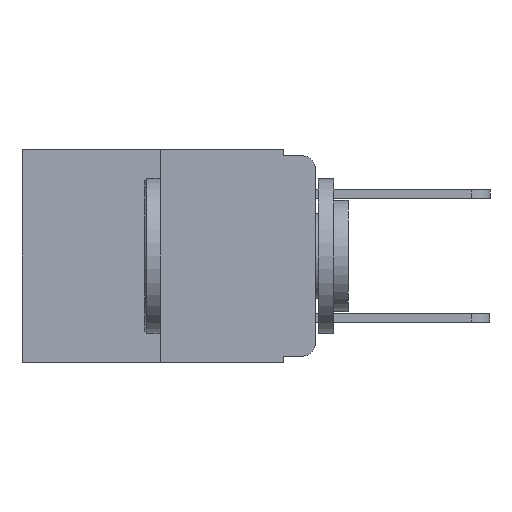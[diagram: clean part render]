
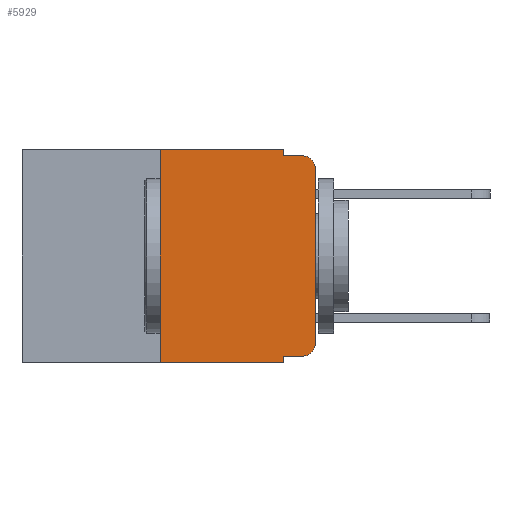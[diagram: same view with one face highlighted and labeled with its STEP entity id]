
A CAD part, left-side view. The second image highlights one B-rep face of the part: STEP entity #5929.
In plain terms, the highlighted planar face has unit normal (-1, 0, 0).
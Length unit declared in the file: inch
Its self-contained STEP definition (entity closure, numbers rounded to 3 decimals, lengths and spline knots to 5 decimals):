
#421 = EDGE_CURVE ( 'NONE', #12266, #12608, #3539, .T. ) ;
#1269 = CIRCLE ( 'NONE', #4434, 0.02 ) ;
#1319 = EDGE_CURVE ( 'NONE', #3115, #10111, #10894, .T. ) ;
#1534 = CARTESIAN_POINT ( 'NONE',  ( 0., 0.02, -0.01 ) ) ;
#1703 = VERTEX_POINT ( 'NONE', #7854 ) ;
#1953 = VECTOR ( 'NONE', #9794, 39.37008 ) ;
#2474 = DIRECTION ( 'NONE',  ( 0., 0., 1. ) ) ;
#2900 = CARTESIAN_POINT ( 'NONE',  ( 0., 0.25, -0.343 ) ) ;
#3115 = VERTEX_POINT ( 'NONE', #11257 ) ;
#3539 = LINE ( 'NONE', #11785, #9305 ) ;
#4050 = CARTESIAN_POINT ( 'NONE',  ( 0., 0.051, -0.333 ) ) ;
#4121 = VECTOR ( 'NONE', #14405, 39.37008 ) ;
#4192 = VERTEX_POINT ( 'NONE', #7693 ) ;
#4434 = AXIS2_PLACEMENT_3D ( 'NONE', #6604, #14104, #13889 ) ;
#4486 = EDGE_CURVE ( 'NONE', #14955, #12266, #11818, .T. ) ;
#5075 = DIRECTION ( 'NONE',  ( 0., 0., -1. ) ) ;
#5216 = EDGE_CURVE ( 'NONE', #6627, #4192, #1269, .T. ) ;
#5263 = EDGE_CURVE ( 'NONE', #14955, #1703, #9962, .T. ) ;
#5427 = DIRECTION ( 'NONE',  ( 0., -1., 0. ) ) ;
#5702 = LINE ( 'NONE', #11659, #8045 ) ;
#5869 = EDGE_CURVE ( 'NONE', #12608, #3115, #8305, .T. ) ;
#5929 = ADVANCED_FACE ( 'NONE', ( #10449 ), #9889, .F. ) ;
#6332 = CIRCLE ( 'NONE', #6473, 0.02 ) ;
#6473 = AXIS2_PLACEMENT_3D ( 'NONE', #7149, #14585, #8295 ) ;
#6604 = CARTESIAN_POINT ( 'NONE',  ( 0., 0.02, -0.313 ) ) ;
#6627 = VERTEX_POINT ( 'NONE', #7120 ) ;
#6712 = CARTESIAN_POINT ( 'NONE',  ( 0., 0.473, -0.343 ) ) ;
#7092 = CARTESIAN_POINT ( 'NONE',  ( 0., 0.25, 0. ) ) ;
#7120 = CARTESIAN_POINT ( 'NONE',  ( 0., 0.02, -0.333 ) ) ;
#7149 = CARTESIAN_POINT ( 'NONE',  ( 0., 0.02, -0.03 ) ) ;
#7528 = CARTESIAN_POINT ( 'NONE',  ( 0., 0.473, 0. ) ) ;
#7693 = CARTESIAN_POINT ( 'NONE',  ( 0., 0., -0.313 ) ) ;
#7854 = CARTESIAN_POINT ( 'NONE',  ( 0., 0.051, -0.343 ) ) ;
#7859 = DIRECTION ( 'NONE',  ( 0., -1., 0. ) ) ;
#8045 = VECTOR ( 'NONE', #5075, 39.37008 ) ;
#8229 = EDGE_CURVE ( 'NONE', #4192, #14223, #12916, .T. ) ;
#8295 = DIRECTION ( 'NONE',  ( 0., 0., -1. ) ) ;
#8305 = LINE ( 'NONE', #13317, #1953 ) ;
#8575 = DIRECTION ( 'NONE',  ( 0., -1., 0. ) ) ;
#8607 = CARTESIAN_POINT ( 'NONE',  ( 0., 0.051, -0.01 ) ) ;
#8660 = VECTOR ( 'NONE', #2474, 39.37008 ) ;
#8827 = CARTESIAN_POINT ( 'NONE',  ( 0., 0.051, -0.333 ) ) ;
#9305 = VECTOR ( 'NONE', #5427, 39.37008 ) ;
#9314 = ORIENTED_EDGE ( 'NONE', *, *, #8229, .T. ) ;
#9353 = VECTOR ( 'NONE', #14069, 39.37008 ) ;
#9794 = DIRECTION ( 'NONE',  ( 0., 0., -1. ) ) ;
#9889 = PLANE ( 'NONE',  #14348 ) ;
#9961 = EDGE_CURVE ( 'NONE', #14886, #1703, #5702, .T. ) ;
#9962 = LINE ( 'NONE', #6712, #12493 ) ;
#10006 = CARTESIAN_POINT ( 'NONE',  ( 0., 0.25, 0. ) ) ;
#10054 = ORIENTED_EDGE ( 'NONE', *, *, #13132, .T. ) ;
#10107 = ORIENTED_EDGE ( 'NONE', *, *, #1319, .F. ) ;
#10111 = VERTEX_POINT ( 'NONE', #1534 ) ;
#10449 = FACE_OUTER_BOUND ( 'NONE', #10638, .T. ) ;
#10560 = VECTOR ( 'NONE', #8575, 39.37008 ) ;
#10638 = EDGE_LOOP ( 'NONE', ( #9314, #10054, #10107, #11231, #11241, #11255, #11309, #11341, #11711, #11885 ) ) ;
#10894 = LINE ( 'NONE', #8607, #10560 ) ;
#11231 = ORIENTED_EDGE ( 'NONE', *, *, #5869, .F. ) ;
#11241 = ORIENTED_EDGE ( 'NONE', *, *, #421, .F. ) ;
#11255 = ORIENTED_EDGE ( 'NONE', *, *, #4486, .F. ) ;
#11257 = CARTESIAN_POINT ( 'NONE',  ( 0., 0.051, -0.01 ) ) ;
#11309 = ORIENTED_EDGE ( 'NONE', *, *, #5263, .T. ) ;
#11341 = ORIENTED_EDGE ( 'NONE', *, *, #9961, .F. ) ;
#11502 = CARTESIAN_POINT ( 'NONE',  ( 0., 0.051, 0. ) ) ;
#11659 = CARTESIAN_POINT ( 'NONE',  ( 0., 0.051, 0. ) ) ;
#11711 = ORIENTED_EDGE ( 'NONE', *, *, #12145, .T. ) ;
#11785 = CARTESIAN_POINT ( 'NONE',  ( 0., 0.473, 0. ) ) ;
#11818 = LINE ( 'NONE', #7092, #8660 ) ;
#11885 = ORIENTED_EDGE ( 'NONE', *, *, #5216, .T. ) ;
#12145 = EDGE_CURVE ( 'NONE', #14886, #6627, #12832, .T. ) ;
#12266 = VERTEX_POINT ( 'NONE', #10006 ) ;
#12493 = VECTOR ( 'NONE', #7859, 39.37008 ) ;
#12608 = VERTEX_POINT ( 'NONE', #11502 ) ;
#12832 = LINE ( 'NONE', #8827, #9353 ) ;
#12916 = LINE ( 'NONE', #14358, #4121 ) ;
#13132 = EDGE_CURVE ( 'NONE', #14223, #10111, #6332, .T. ) ;
#13317 = CARTESIAN_POINT ( 'NONE',  ( 0., 0.051, 0. ) ) ;
#13889 = DIRECTION ( 'NONE',  ( 0., 0., -1. ) ) ;
#14069 = DIRECTION ( 'NONE',  ( 0., -1., 0. ) ) ;
#14102 = CARTESIAN_POINT ( 'NONE',  ( 0., 0., -0.03 ) ) ;
#14104 = DIRECTION ( 'NONE',  ( -1., 0., 0. ) ) ;
#14223 = VERTEX_POINT ( 'NONE', #14102 ) ;
#14348 = AXIS2_PLACEMENT_3D ( 'NONE', #7528, #14509, #14403 ) ;
#14358 = CARTESIAN_POINT ( 'NONE',  ( 0., 0., 0. ) ) ;
#14403 = DIRECTION ( 'NONE',  ( 0., 0., -1. ) ) ;
#14405 = DIRECTION ( 'NONE',  ( 0., 0., 1. ) ) ;
#14509 = DIRECTION ( 'NONE',  ( 1., 0., 0. ) ) ;
#14585 = DIRECTION ( 'NONE',  ( -1., 0., 0. ) ) ;
#14886 = VERTEX_POINT ( 'NONE', #4050 ) ;
#14955 = VERTEX_POINT ( 'NONE', #2900 ) ;
